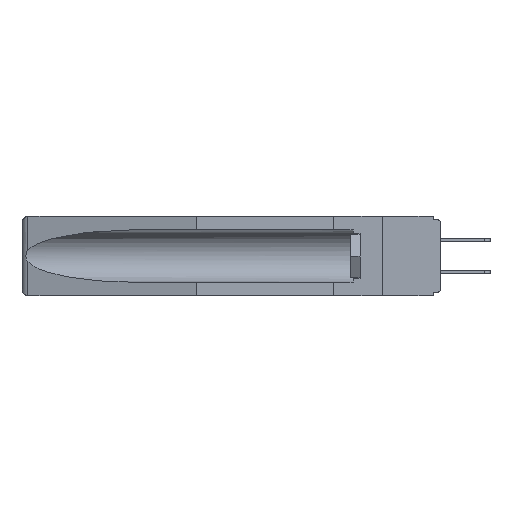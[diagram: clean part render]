
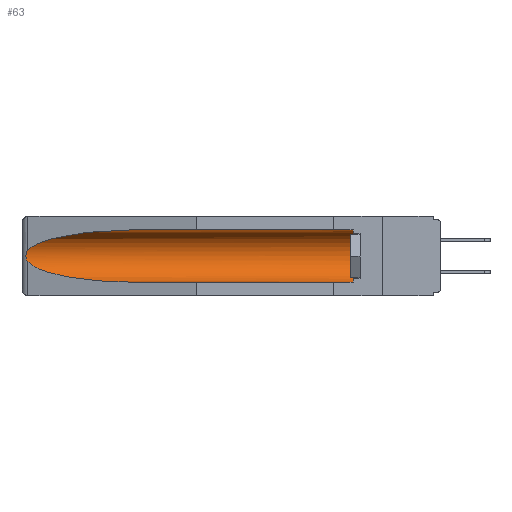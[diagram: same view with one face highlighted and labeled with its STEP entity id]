
A CAD part, left-side view. The second image highlights one B-rep face of the part: STEP entity #63.
In plain terms, the highlighted cylindrical face has radius 2.857 mm (diameter 5.715 mm), a partial arc.
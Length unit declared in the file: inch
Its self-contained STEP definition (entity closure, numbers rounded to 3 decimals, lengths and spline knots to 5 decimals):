
#4 = DIRECTION ( 'NONE',  ( 0., -1., 0. ) ) ;
#63 = ADVANCED_FACE ( 'NONE', ( #15714 ), #5385, .F. ) ;
#381 = CARTESIAN_POINT ( 'NONE',  ( 0.26537, 1.52718, -0.19328 ) ) ;
#639 = EDGE_CURVE ( 'NONE', #14322, #8157, #2007, .T. ) ;
#1275 = EDGE_CURVE ( 'NONE', #10960, #14412, #19438, .T. ) ;
#1276 = ORIENTED_EDGE ( 'NONE', *, *, #1275, .T. ) ;
#1515 = VECTOR ( 'NONE', #12518, 39.37008 ) ;
#2007 =( BOUNDED_CURVE ( )  B_SPLINE_CURVE ( 3, ( #11488, #13100, #2447, #2186 ),
 .UNSPECIFIED., .F., .F. ) 
 B_SPLINE_CURVE_WITH_KNOTS ( ( 4, 4 ),
 ( 0.1948, 1.5708 ),
 .UNSPECIFIED. ) 
 CURVE ( )  GEOMETRIC_REPRESENTATION_ITEM ( )  RATIONAL_B_SPLINE_CURVE ( ( 1., 0.848, 0.848, 1. ) ) 
 REPRESENTATION_ITEM ( '' )  );
#2099 = ORIENTED_EDGE ( 'NONE', *, *, #5417, .T. ) ;
#2186 = CARTESIAN_POINT ( 'NONE',  ( 0.155, 1.07973, -0.284 ) ) ;
#2379 = AXIS2_PLACEMENT_3D ( 'NONE', #15617, #9517, #3724 ) ;
#2447 = CARTESIAN_POINT ( 'NONE',  ( 0.21114, 1.30732, -0.284 ) ) ;
#3558 = CARTESIAN_POINT ( 'NONE',  ( 0.2673, 1.53269, -0.17917 ) ) ;
#3724 = DIRECTION ( 'NONE',  ( 0., 0., 1. ) ) ;
#3971 = EDGE_CURVE ( 'NONE', #10960, #8157, #9473, .T. ) ;
#4354 = CARTESIAN_POINT ( 'NONE',  ( 0.155, 0.126, -0.059 ) ) ;
#4963 = CARTESIAN_POINT ( 'NONE',  ( 0.2675, 1.53308, -0.16763 ) ) ;
#5385 = CYLINDRICAL_SURFACE ( 'NONE', #2379, 0.1125 ) ;
#5417 = EDGE_CURVE ( 'NONE', #17691, #14322, #6795, .T. ) ;
#5713 = EDGE_CURVE ( 'NONE', #18868, #17691, #14222, .T. ) ;
#6071 = CARTESIAN_POINT ( 'NONE',  ( 0.155, 0.126, -0.284 ) ) ;
#6268 = CARTESIAN_POINT ( 'NONE',  ( 0.155, 1.07973, -0.059 ) ) ;
#6554 = CARTESIAN_POINT ( 'NONE',  ( 0.26537, 1.52718, -0.14972 ) ) ;
#6795 = B_SPLINE_CURVE_WITH_KNOTS ( 'NONE', 3,
 ( #6554, #15774, #11111, #9623, #4963, #11235, #3558, #9551, #17325, #381 ),
 .UNSPECIFIED., .F., .F.,
 ( 4, 2, 2, 2, 4 ),
 ( 0., 0.00029, 0.00058, 0.00087, 0.00117 ),
 .UNSPECIFIED. ) ;
#6843 = ORIENTED_EDGE ( 'NONE', *, *, #3971, .F. ) ;
#6994 = ORIENTED_EDGE ( 'NONE', *, *, #639, .T. ) ;
#8025 = LINE ( 'NONE', #13730, #14756 ) ;
#8157 = VERTEX_POINT ( 'NONE', #18898 ) ;
#8772 = CARTESIAN_POINT ( 'NONE',  ( 0.25451, 1.48313, -0.09465 ) ) ;
#9418 = CARTESIAN_POINT ( 'NONE',  ( 0.155, -0.30754, -0.284 ) ) ;
#9473 = LINE ( 'NONE', #9418, #1515 ) ;
#9497 = CARTESIAN_POINT ( 'NONE',  ( 0.26537, 1.52718, -0.14972 ) ) ;
#9517 = DIRECTION ( 'NONE',  ( 0., 1., 0. ) ) ;
#9551 = CARTESIAN_POINT ( 'NONE',  ( 0.26655, 1.53094, -0.18657 ) ) ;
#9623 = CARTESIAN_POINT ( 'NONE',  ( 0.2673, 1.5327, -0.16383 ) ) ;
#10148 = CARTESIAN_POINT ( 'NONE',  ( 0.26537, 1.52718, -0.14972 ) ) ;
#10960 = VERTEX_POINT ( 'NONE', #6071 ) ;
#11111 = CARTESIAN_POINT ( 'NONE',  ( 0.26654, 1.53092, -0.15636 ) ) ;
#11235 = CARTESIAN_POINT ( 'NONE',  ( 0.2675, 1.53308, -0.17534 ) ) ;
#11488 = CARTESIAN_POINT ( 'NONE',  ( 0.26537, 1.52718, -0.19328 ) ) ;
#11610 = EDGE_LOOP ( 'NONE', ( #12159, #2099, #6994, #6843, #1276, #16405 ) ) ;
#12159 = ORIENTED_EDGE ( 'NONE', *, *, #5713, .T. ) ;
#12518 = DIRECTION ( 'NONE',  ( 0., 1., 0. ) ) ;
#13100 = CARTESIAN_POINT ( 'NONE',  ( 0.25451, 1.48313, -0.24835 ) ) ;
#13730 = CARTESIAN_POINT ( 'NONE',  ( 0.155, -0.30754, -0.059 ) ) ;
#14025 = EDGE_CURVE ( 'NONE', #14412, #18868, #8025, .T. ) ;
#14222 =( BOUNDED_CURVE ( )  B_SPLINE_CURVE ( 3, ( #14907, #16298, #8772, #10148 ),
 .UNSPECIFIED., .F., .F. ) 
 B_SPLINE_CURVE_WITH_KNOTS ( ( 4, 4 ),
 ( 4.71239, 6.08839 ),
 .UNSPECIFIED. ) 
 CURVE ( )  GEOMETRIC_REPRESENTATION_ITEM ( )  RATIONAL_B_SPLINE_CURVE ( ( 1., 0.848, 0.848, 1. ) ) 
 REPRESENTATION_ITEM ( '' )  );
#14322 = VERTEX_POINT ( 'NONE', #19045 ) ;
#14412 = VERTEX_POINT ( 'NONE', #4354 ) ;
#14756 = VECTOR ( 'NONE', #17010, 39.37008 ) ;
#14907 = CARTESIAN_POINT ( 'NONE',  ( 0.155, 1.07973, -0.059 ) ) ;
#15617 = CARTESIAN_POINT ( 'NONE',  ( 0.155, -0.30754, -0.1715 ) ) ;
#15651 = AXIS2_PLACEMENT_3D ( 'NONE', #16728, #4, #18244 ) ;
#15714 = FACE_OUTER_BOUND ( 'NONE', #11610, .T. ) ;
#15774 = CARTESIAN_POINT ( 'NONE',  ( 0.26597, 1.52961, -0.15275 ) ) ;
#16298 = CARTESIAN_POINT ( 'NONE',  ( 0.21114, 1.30732, -0.059 ) ) ;
#16405 = ORIENTED_EDGE ( 'NONE', *, *, #14025, .T. ) ;
#16728 = CARTESIAN_POINT ( 'NONE',  ( 0.155, 0.126, -0.1715 ) ) ;
#17010 = DIRECTION ( 'NONE',  ( 0., 1., 0. ) ) ;
#17325 = CARTESIAN_POINT ( 'NONE',  ( 0.26597, 1.5296, -0.19026 ) ) ;
#17691 = VERTEX_POINT ( 'NONE', #9497 ) ;
#18244 = DIRECTION ( 'NONE',  ( 0., 0., 1. ) ) ;
#18868 = VERTEX_POINT ( 'NONE', #6268 ) ;
#18898 = CARTESIAN_POINT ( 'NONE',  ( 0.155, 1.07973, -0.284 ) ) ;
#19045 = CARTESIAN_POINT ( 'NONE',  ( 0.26537, 1.52718, -0.19328 ) ) ;
#19438 = CIRCLE ( 'NONE', #15651, 0.1125 ) ;
